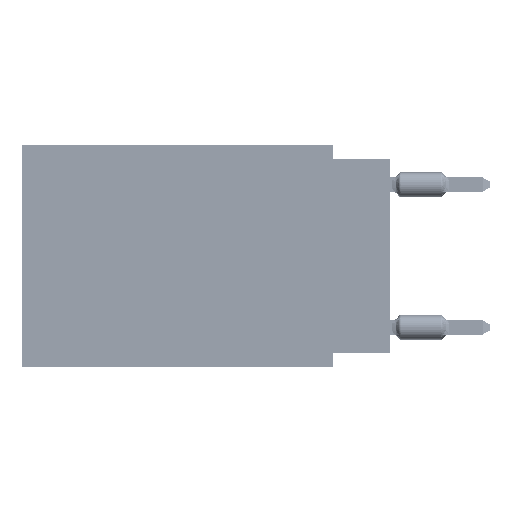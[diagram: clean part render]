
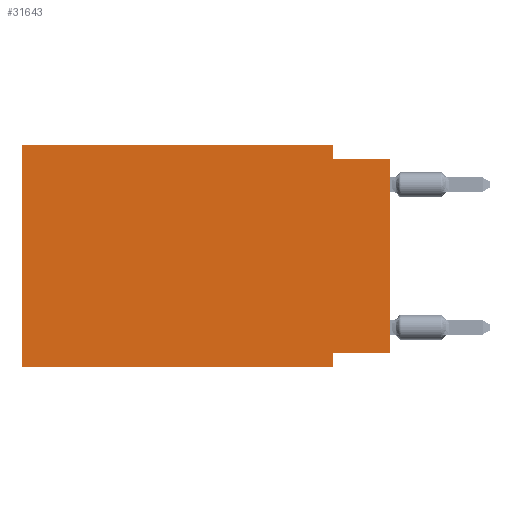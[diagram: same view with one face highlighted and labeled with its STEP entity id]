
A CAD part, left-side view. The second image highlights one B-rep face of the part: STEP entity #31643.
In plain terms, the highlighted planar face has unit normal (-1, 0, 0).
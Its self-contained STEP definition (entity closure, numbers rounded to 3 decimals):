
#347 = DIRECTION ( 'NONE',  ( 0., 0., 1. ) ) ;
#1703 = DIRECTION ( 'NONE',  ( 0., -1., 0. ) ) ;
#3531 = LINE ( 'NONE', #16698, #34149 ) ;
#4478 = CARTESIAN_POINT ( 'NONE',  ( 0., 0., -9.271 ) ) ;
#5323 = CARTESIAN_POINT ( 'NONE',  ( 0., 16.383, 0. ) ) ;
#13415 = CARTESIAN_POINT ( 'NONE',  ( 0., 0., -0.635 ) ) ;
#14875 = LINE ( 'NONE', #70305, #25554 ) ;
#16547 = EDGE_CURVE ( 'NONE', #60518, #31503, #42274, .T. ) ;
#16698 = CARTESIAN_POINT ( 'NONE',  ( 0., 16.383, 0. ) ) ;
#16874 = VERTEX_POINT ( 'NONE', #13415 ) ;
#18818 = VERTEX_POINT ( 'NONE', #44304 ) ;
#19455 = ORIENTED_EDGE ( 'NONE', *, *, #56988, .F. ) ;
#22021 = CARTESIAN_POINT ( 'NONE',  ( 0., 16.383, -9.906 ) ) ;
#23815 = EDGE_CURVE ( 'NONE', #45111, #16874, #59424, .T. ) ;
#24094 = DIRECTION ( 'NONE',  ( 1., 0., 0. ) ) ;
#25554 = VECTOR ( 'NONE', #1703, 1000. ) ;
#26787 = VERTEX_POINT ( 'NONE', #64212 ) ;
#28833 = DIRECTION ( 'NONE',  ( 0., 1., 0. ) ) ;
#30087 = ORIENTED_EDGE ( 'NONE', *, *, #66240, .F. ) ;
#31503 = VERTEX_POINT ( 'NONE', #33713 ) ;
#31643 = ADVANCED_FACE ( 'NONE', ( #72350 ), #36454, .F. ) ;
#33713 = CARTESIAN_POINT ( 'NONE',  ( 0., 16.383, 0. ) ) ;
#34149 = VECTOR ( 'NONE', #41042, 1000. ) ;
#35215 = LINE ( 'NONE', #4478, #47808 ) ;
#36454 = PLANE ( 'NONE',  #56919 ) ;
#36999 = VERTEX_POINT ( 'NONE', #48432 ) ;
#38300 = CARTESIAN_POINT ( 'NONE',  ( 0., 2.54, 0. ) ) ;
#39249 = ORIENTED_EDGE ( 'NONE', *, *, #66636, .F. ) ;
#41042 = DIRECTION ( 'NONE',  ( 0., -1., 0. ) ) ;
#42274 = LINE ( 'NONE', #73752, #59973 ) ;
#43338 = DIRECTION ( 'NONE',  ( 0., 0., -1. ) ) ;
#43989 = EDGE_CURVE ( 'NONE', #60518, #26787, #77039, .T. ) ;
#44304 = CARTESIAN_POINT ( 'NONE',  ( 0., 2.54, -0.635 ) ) ;
#44906 = CARTESIAN_POINT ( 'NONE',  ( 0., 2.54, -9.906 ) ) ;
#45111 = VERTEX_POINT ( 'NONE', #76277 ) ;
#47130 = VECTOR ( 'NONE', #51066, 1000. ) ;
#47808 = VECTOR ( 'NONE', #28833, 1000. ) ;
#48004 = VECTOR ( 'NONE', #51953, 1000. ) ;
#48423 = DIRECTION ( 'NONE',  ( 0., 0., -1. ) ) ;
#48432 = CARTESIAN_POINT ( 'NONE',  ( 0., 2.54, -9.271 ) ) ;
#51066 = DIRECTION ( 'NONE',  ( 0., 0., -1. ) ) ;
#51953 = DIRECTION ( 'NONE',  ( 0., -1., 0. ) ) ;
#53938 = ORIENTED_EDGE ( 'NONE', *, *, #58840, .F. ) ;
#56919 = AXIS2_PLACEMENT_3D ( 'NONE', #5323, #24094, #48423 ) ;
#56988 = EDGE_CURVE ( 'NONE', #31503, #76117, #3531, .T. ) ;
#58840 = EDGE_CURVE ( 'NONE', #18818, #16874, #14875, .T. ) ;
#59033 = DIRECTION ( 'NONE',  ( 0., 0., 1. ) ) ;
#59424 = LINE ( 'NONE', #65006, #61725 ) ;
#59973 = VECTOR ( 'NONE', #347, 1000. ) ;
#60518 = VERTEX_POINT ( 'NONE', #71072 ) ;
#61725 = VECTOR ( 'NONE', #59033, 1000. ) ;
#63020 = ORIENTED_EDGE ( 'NONE', *, *, #16547, .F. ) ;
#63637 = ORIENTED_EDGE ( 'NONE', *, *, #71545, .F. ) ;
#63787 = CARTESIAN_POINT ( 'NONE',  ( 0., 2.54, 0. ) ) ;
#64212 = CARTESIAN_POINT ( 'NONE',  ( 0., 2.54, -9.906 ) ) ;
#65006 = CARTESIAN_POINT ( 'NONE',  ( 0., 0., 0. ) ) ;
#66240 = EDGE_CURVE ( 'NONE', #45111, #36999, #35215, .T. ) ;
#66636 = EDGE_CURVE ( 'NONE', #36999, #26787, #75199, .T. ) ;
#66929 = VECTOR ( 'NONE', #43338, 1000. ) ;
#67444 = LINE ( 'NONE', #38300, #47130 ) ;
#69850 = ORIENTED_EDGE ( 'NONE', *, *, #23815, .T. ) ;
#70305 = CARTESIAN_POINT ( 'NONE',  ( 0., 0., -0.635 ) ) ;
#70745 = EDGE_LOOP ( 'NONE', ( #69850, #53938, #63637, #19455, #63020, #72941, #39249, #30087 ) ) ;
#71072 = CARTESIAN_POINT ( 'NONE',  ( 0., 16.383, -9.906 ) ) ;
#71545 = EDGE_CURVE ( 'NONE', #76117, #18818, #67444, .T. ) ;
#72350 = FACE_OUTER_BOUND ( 'NONE', #70745, .T. ) ;
#72941 = ORIENTED_EDGE ( 'NONE', *, *, #43989, .T. ) ;
#73752 = CARTESIAN_POINT ( 'NONE',  ( 0., 16.383, 0. ) ) ;
#75199 = LINE ( 'NONE', #44906, #66929 ) ;
#76117 = VERTEX_POINT ( 'NONE', #63787 ) ;
#76277 = CARTESIAN_POINT ( 'NONE',  ( 0., 0., -9.271 ) ) ;
#77039 = LINE ( 'NONE', #22021, #48004 ) ;
